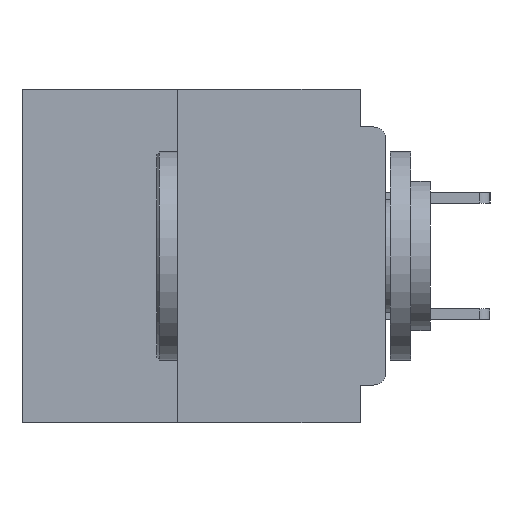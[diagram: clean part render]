
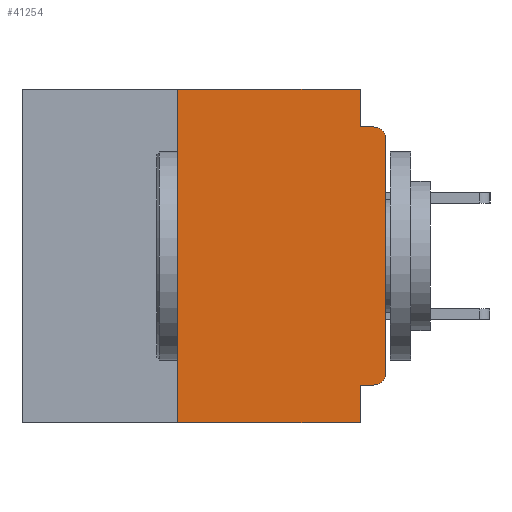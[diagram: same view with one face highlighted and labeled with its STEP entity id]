
A CAD part, left-side view. The second image highlights one B-rep face of the part: STEP entity #41254.
In plain terms, the highlighted planar face has unit normal (-1, 0, 0).
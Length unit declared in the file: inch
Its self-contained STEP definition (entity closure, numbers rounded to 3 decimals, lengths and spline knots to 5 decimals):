
#1050 = CARTESIAN_POINT ( 'NONE',  ( 0., 0.437, -0.4 ) ) ;
#1095 = VERTEX_POINT ( 'NONE', #45611 ) ;
#1338 = ORIENTED_EDGE ( 'NONE', *, *, #59794, .F. ) ;
#3614 = VECTOR ( 'NONE', #31142, 39.37008 ) ;
#4876 = CARTESIAN_POINT ( 'NONE',  ( 0., 0.031, -0.355 ) ) ;
#5088 = VECTOR ( 'NONE', #28013, 39.37008 ) ;
#5707 = VERTEX_POINT ( 'NONE', #18768 ) ;
#5892 = CARTESIAN_POINT ( 'NONE',  ( 0., 0., -0.34 ) ) ;
#8288 = ORIENTED_EDGE ( 'NONE', *, *, #32040, .F. ) ;
#8705 = VERTEX_POINT ( 'NONE', #4876 ) ;
#9875 = VECTOR ( 'NONE', #15500, 39.37008 ) ;
#10223 = AXIS2_PLACEMENT_3D ( 'NONE', #20652, #53811, #25451 ) ;
#10287 = EDGE_LOOP ( 'NONE', ( #27001, #21649, #24065, #55293, #1338, #22673, #27252, #24581, #8288, #54062 ) ) ;
#10308 = CARTESIAN_POINT ( 'NONE',  ( 0., 0.031, -0.045 ) ) ;
#10626 = CARTESIAN_POINT ( 'NONE',  ( 0., 0., 0. ) ) ;
#13232 = CARTESIAN_POINT ( 'NONE',  ( 0., 0.437, 0. ) ) ;
#13589 = FACE_OUTER_BOUND ( 'NONE', #10287, .T. ) ;
#14171 = VECTOR ( 'NONE', #34449, 39.37008 ) ;
#14843 = CARTESIAN_POINT ( 'NONE',  ( 0., 0.015, -0.34 ) ) ;
#15500 = DIRECTION ( 'NONE',  ( 0., 0., 1. ) ) ;
#16386 = LINE ( 'NONE', #21507, #3614 ) ;
#17241 = EDGE_CURVE ( 'NONE', #45757, #25342, #24455, .T. ) ;
#17882 = VECTOR ( 'NONE', #43161, 39.37008 ) ;
#18768 = CARTESIAN_POINT ( 'NONE',  ( 0., 0.25, -0.4 ) ) ;
#19153 = AXIS2_PLACEMENT_3D ( 'NONE', #13232, #60740, #32442 ) ;
#19348 = LINE ( 'NONE', #42097, #5088 ) ;
#19633 = DIRECTION ( 'NONE',  ( 0., 0., -1. ) ) ;
#20652 = CARTESIAN_POINT ( 'NONE',  ( 0., 0.015, -0.06 ) ) ;
#20921 = EDGE_CURVE ( 'NONE', #25342, #58619, #35271, .T. ) ;
#21507 = CARTESIAN_POINT ( 'NONE',  ( 0., 0., -0.355 ) ) ;
#21649 = ORIENTED_EDGE ( 'NONE', *, *, #39562, .T. ) ;
#22673 = ORIENTED_EDGE ( 'NONE', *, *, #57225, .F. ) ;
#23934 = CARTESIAN_POINT ( 'NONE',  ( 0., 0.437, 0. ) ) ;
#24065 = ORIENTED_EDGE ( 'NONE', *, *, #27672, .F. ) ;
#24322 = EDGE_CURVE ( 'NONE', #41319, #54171, #47971, .T. ) ;
#24455 = CIRCLE ( 'NONE', #40037, 0.015 ) ;
#24581 = ORIENTED_EDGE ( 'NONE', *, *, #28714, .F. ) ;
#25342 = VERTEX_POINT ( 'NONE', #5892 ) ;
#25451 = DIRECTION ( 'NONE',  ( 0., 0., -1. ) ) ;
#26849 = LINE ( 'NONE', #1050, #14171 ) ;
#27001 = ORIENTED_EDGE ( 'NONE', *, *, #20921, .T. ) ;
#27252 = ORIENTED_EDGE ( 'NONE', *, *, #31883, .T. ) ;
#27659 = PLANE ( 'NONE',  #19153 ) ;
#27672 = EDGE_CURVE ( 'NONE', #54171, #51900, #30589, .T. ) ;
#28013 = DIRECTION ( 'NONE',  ( 0., 0., 1. ) ) ;
#28714 = EDGE_CURVE ( 'NONE', #8705, #36941, #43067, .T. ) ;
#28758 = DIRECTION ( 'NONE',  ( 0., -1., 0. ) ) ;
#28910 = CARTESIAN_POINT ( 'NONE',  ( 0., 0., -0.06 ) ) ;
#30589 = LINE ( 'NONE', #38378, #17882 ) ;
#30872 = CARTESIAN_POINT ( 'NONE',  ( 0., 0.015, -0.045 ) ) ;
#31142 = DIRECTION ( 'NONE',  ( 0., 1., 0. ) ) ;
#31145 = CARTESIAN_POINT ( 'NONE',  ( 0., 0.015, -0.355 ) ) ;
#31883 = EDGE_CURVE ( 'NONE', #5707, #36941, #26849, .T. ) ;
#32040 = EDGE_CURVE ( 'NONE', #45757, #8705, #16386, .T. ) ;
#32442 = DIRECTION ( 'NONE',  ( 0., 0., -1. ) ) ;
#34449 = DIRECTION ( 'NONE',  ( 0., -1., 0. ) ) ;
#35271 = LINE ( 'NONE', #10626, #9875 ) ;
#35343 = VECTOR ( 'NONE', #38763, 39.37008 ) ;
#36941 = VERTEX_POINT ( 'NONE', #52664 ) ;
#38378 = CARTESIAN_POINT ( 'NONE',  ( 0., 0., -0.045 ) ) ;
#38763 = DIRECTION ( 'NONE',  ( 0., 0., -1. ) ) ;
#39562 = EDGE_CURVE ( 'NONE', #58619, #51900, #59842, .T. ) ;
#40037 = AXIS2_PLACEMENT_3D ( 'NONE', #14843, #48093, #19633 ) ;
#41254 = ADVANCED_FACE ( 'NONE', ( #13589 ), #27659, .F. ) ;
#41319 = VERTEX_POINT ( 'NONE', #60930 ) ;
#41545 = VECTOR ( 'NONE', #54353, 39.37008 ) ;
#42097 = CARTESIAN_POINT ( 'NONE',  ( 0., 0.25, -0.4 ) ) ;
#43067 = LINE ( 'NONE', #45098, #41545 ) ;
#43161 = DIRECTION ( 'NONE',  ( 0., -1., 0. ) ) ;
#45098 = CARTESIAN_POINT ( 'NONE',  ( 0., 0.031, -0.4 ) ) ;
#45611 = CARTESIAN_POINT ( 'NONE',  ( 0., 0.25, 0. ) ) ;
#45757 = VERTEX_POINT ( 'NONE', #31145 ) ;
#47971 = LINE ( 'NONE', #48116, #35343 ) ;
#48093 = DIRECTION ( 'NONE',  ( -1., 0., 0. ) ) ;
#48116 = CARTESIAN_POINT ( 'NONE',  ( 0., 0.031, 0. ) ) ;
#48713 = LINE ( 'NONE', #23934, #56824 ) ;
#51900 = VERTEX_POINT ( 'NONE', #30872 ) ;
#52664 = CARTESIAN_POINT ( 'NONE',  ( 0., 0.031, -0.4 ) ) ;
#53811 = DIRECTION ( 'NONE',  ( -1., 0., 0. ) ) ;
#54062 = ORIENTED_EDGE ( 'NONE', *, *, #17241, .T. ) ;
#54171 = VERTEX_POINT ( 'NONE', #10308 ) ;
#54353 = DIRECTION ( 'NONE',  ( 0., 0., -1. ) ) ;
#55293 = ORIENTED_EDGE ( 'NONE', *, *, #24322, .F. ) ;
#56824 = VECTOR ( 'NONE', #28758, 39.37008 ) ;
#57225 = EDGE_CURVE ( 'NONE', #5707, #1095, #19348, .T. ) ;
#58619 = VERTEX_POINT ( 'NONE', #28910 ) ;
#59794 = EDGE_CURVE ( 'NONE', #1095, #41319, #48713, .T. ) ;
#59842 = CIRCLE ( 'NONE', #10223, 0.015 ) ;
#60740 = DIRECTION ( 'NONE',  ( 1., 0., 0. ) ) ;
#60930 = CARTESIAN_POINT ( 'NONE',  ( 0., 0.031, 0. ) ) ;
